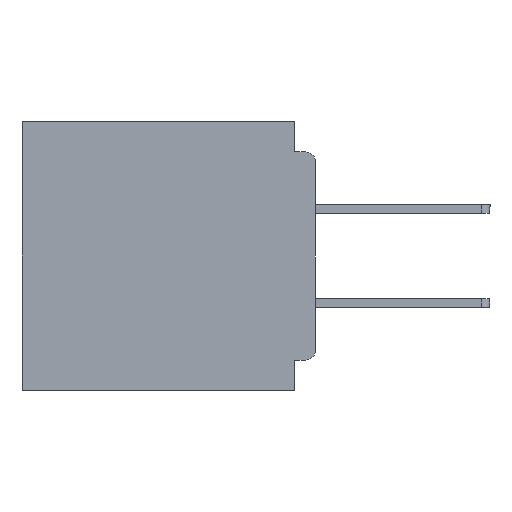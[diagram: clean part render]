
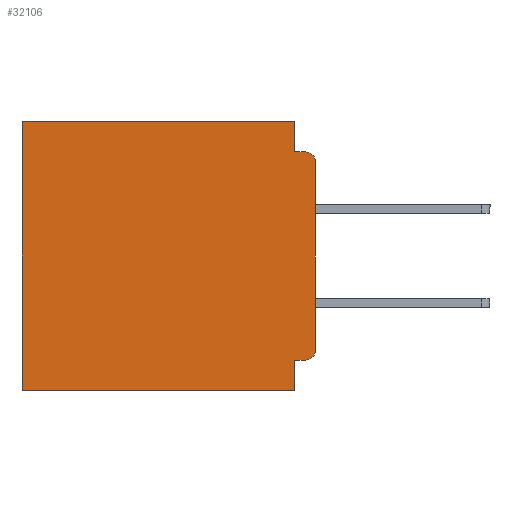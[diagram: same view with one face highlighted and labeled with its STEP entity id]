
A CAD part, left-side view. The second image highlights one B-rep face of the part: STEP entity #32106.
In plain terms, the highlighted planar face has unit normal (-1, 0, 0).
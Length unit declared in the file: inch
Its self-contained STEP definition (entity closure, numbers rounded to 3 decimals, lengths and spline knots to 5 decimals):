
#541 = LINE ( 'NONE', #1973, #42620 ) ;
#576 = EDGE_CURVE ( 'NONE', #24921, #27459, #48411, .T. ) ;
#1276 = VERTEX_POINT ( 'NONE', #49345 ) ;
#1973 = CARTESIAN_POINT ( 'NONE',  ( 0.3, 0., -0.4 ) ) ;
#2923 = ORIENTED_EDGE ( 'NONE', *, *, #19662, .F. ) ;
#3037 = ORIENTED_EDGE ( 'NONE', *, *, #3956, .F. ) ;
#3356 = EDGE_CURVE ( 'NONE', #4445, #14163, #34812, .T. ) ;
#3956 = EDGE_CURVE ( 'NONE', #1276, #4445, #29619, .T. ) ;
#4445 = VERTEX_POINT ( 'NONE', #17916 ) ;
#4717 = CARTESIAN_POINT ( 'NONE',  ( 0.3, 0., -0.4 ) ) ;
#5604 = ORIENTED_EDGE ( 'NONE', *, *, #14906, .F. ) ;
#8068 = ORIENTED_EDGE ( 'NONE', *, *, #576, .F. ) ;
#8786 = DIRECTION ( 'NONE',  ( 1., 0., 0. ) ) ;
#9751 = CIRCLE ( 'NONE', #35528, 0.015 ) ;
#9916 = ORIENTED_EDGE ( 'NONE', *, *, #21294, .T. ) ;
#10152 = CARTESIAN_POINT ( 'NONE',  ( 0.3, 0.437, 0. ) ) ;
#10238 = CARTESIAN_POINT ( 'NONE',  ( 0.3, 0.031, -0.4 ) ) ;
#14163 = VERTEX_POINT ( 'NONE', #17513 ) ;
#14285 = ORIENTED_EDGE ( 'NONE', *, *, #16087, .T. ) ;
#14349 = CARTESIAN_POINT ( 'NONE',  ( 0.3, 0., -0.045 ) ) ;
#14906 = EDGE_CURVE ( 'NONE', #37538, #44728, #541, .T. ) ;
#15687 = CARTESIAN_POINT ( 'NONE',  ( 0.3, 0., -0.355 ) ) ;
#15803 = LINE ( 'NONE', #40342, #40226 ) ;
#16087 = EDGE_CURVE ( 'NONE', #18767, #38620, #46026, .T. ) ;
#17513 = CARTESIAN_POINT ( 'NONE',  ( 0.3, 0.015, -0.045 ) ) ;
#17916 = CARTESIAN_POINT ( 'NONE',  ( 0.3, 0.031, -0.045 ) ) ;
#18767 = VERTEX_POINT ( 'NONE', #10152 ) ;
#19227 = CARTESIAN_POINT ( 'NONE',  ( 0.3, 0.015, -0.06 ) ) ;
#19255 = DIRECTION ( 'NONE',  ( 0., 1., 0. ) ) ;
#19662 = EDGE_CURVE ( 'NONE', #27459, #32851, #29667, .T. ) ;
#19992 = DIRECTION ( 'NONE',  ( 0., 1., 0. ) ) ;
#21294 = EDGE_CURVE ( 'NONE', #1276, #18767, #33327, .T. ) ;
#22009 = CARTESIAN_POINT ( 'NONE',  ( 0.3, 0., -0.34 ) ) ;
#22091 = DIRECTION ( 'NONE',  ( 0., 1., 0. ) ) ;
#22133 = CARTESIAN_POINT ( 'NONE',  ( 0.3, 0.437, -0.4 ) ) ;
#22221 = CARTESIAN_POINT ( 'NONE',  ( 0.3, 0.031, -0.355 ) ) ;
#22444 = VECTOR ( 'NONE', #19255, 39.37008 ) ;
#22645 = CARTESIAN_POINT ( 'NONE',  ( 0.3, 0.015, -0.34 ) ) ;
#22954 = CARTESIAN_POINT ( 'NONE',  ( 0.3, 0.031, 0. ) ) ;
#23049 = VECTOR ( 'NONE', #30181, 39.37008 ) ;
#23368 = ORIENTED_EDGE ( 'NONE', *, *, #3356, .F. ) ;
#23937 = VECTOR ( 'NONE', #33295, 39.37008 ) ;
#24040 = DIRECTION ( 'NONE',  ( 0., 0., -1. ) ) ;
#24921 = VERTEX_POINT ( 'NONE', #25912 ) ;
#25865 = ORIENTED_EDGE ( 'NONE', *, *, #41685, .T. ) ;
#25912 = CARTESIAN_POINT ( 'NONE',  ( 0.3, 0.015, -0.355 ) ) ;
#26760 = DIRECTION ( 'NONE',  ( 0., 0., -1. ) ) ;
#27459 = VERTEX_POINT ( 'NONE', #22221 ) ;
#29060 = PLANE ( 'NONE',  #47614 ) ;
#29619 = LINE ( 'NONE', #22954, #37915 ) ;
#29667 = LINE ( 'NONE', #40519, #51283 ) ;
#30181 = DIRECTION ( 'NONE',  ( 0., 0., -1. ) ) ;
#30219 = EDGE_LOOP ( 'NONE', ( #5604, #38073, #23368, #3037, #9916, #14285, #32913, #2923, #8068, #25865 ) ) ;
#32106 = ADVANCED_FACE ( 'NONE', ( #40430 ), #29060, .F. ) ;
#32851 = VERTEX_POINT ( 'NONE', #10238 ) ;
#32913 = ORIENTED_EDGE ( 'NONE', *, *, #40198, .F. ) ;
#33295 = DIRECTION ( 'NONE',  ( 0., -1., 0. ) ) ;
#33327 = LINE ( 'NONE', #39599, #22444 ) ;
#34812 = LINE ( 'NONE', #14349, #23937 ) ;
#35528 = AXIS2_PLACEMENT_3D ( 'NONE', #19227, #47730, #24040 ) ;
#37302 = DIRECTION ( 'NONE',  ( 0., 0., -1. ) ) ;
#37538 = VERTEX_POINT ( 'NONE', #42767 ) ;
#37591 = VECTOR ( 'NONE', #22091, 39.37008 ) ;
#37644 = EDGE_CURVE ( 'NONE', #37538, #14163, #9751, .T. ) ;
#37915 = VECTOR ( 'NONE', #51402, 39.37008 ) ;
#38073 = ORIENTED_EDGE ( 'NONE', *, *, #37644, .T. ) ;
#38620 = VERTEX_POINT ( 'NONE', #45977 ) ;
#38822 = CIRCLE ( 'NONE', #51974, 0.015 ) ;
#39599 = CARTESIAN_POINT ( 'NONE',  ( 0.3, 0., 0. ) ) ;
#40198 = EDGE_CURVE ( 'NONE', #32851, #38620, #15803, .T. ) ;
#40226 = VECTOR ( 'NONE', #19992, 39.37008 ) ;
#40342 = CARTESIAN_POINT ( 'NONE',  ( 0.3, 0., -0.4 ) ) ;
#40430 = FACE_OUTER_BOUND ( 'NONE', #30219, .T. ) ;
#40519 = CARTESIAN_POINT ( 'NONE',  ( 0.3, 0.031, -0.4 ) ) ;
#41685 = EDGE_CURVE ( 'NONE', #24921, #44728, #38822, .T. ) ;
#42620 = VECTOR ( 'NONE', #42747, 39.37008 ) ;
#42747 = DIRECTION ( 'NONE',  ( 0., 0., -1. ) ) ;
#42767 = CARTESIAN_POINT ( 'NONE',  ( 0.3, 0., -0.06 ) ) ;
#44728 = VERTEX_POINT ( 'NONE', #22009 ) ;
#45977 = CARTESIAN_POINT ( 'NONE',  ( 0.3, 0.437, -0.4 ) ) ;
#46026 = LINE ( 'NONE', #22133, #23049 ) ;
#47614 = AXIS2_PLACEMENT_3D ( 'NONE', #4717, #8786, #37302 ) ;
#47730 = DIRECTION ( 'NONE',  ( -1., 0., 0. ) ) ;
#48411 = LINE ( 'NONE', #15687, #37591 ) ;
#49345 = CARTESIAN_POINT ( 'NONE',  ( 0.3, 0.031, 0. ) ) ;
#51095 = DIRECTION ( 'NONE',  ( -1., 0., 0. ) ) ;
#51283 = VECTOR ( 'NONE', #52679, 39.37008 ) ;
#51402 = DIRECTION ( 'NONE',  ( 0., 0., -1. ) ) ;
#51974 = AXIS2_PLACEMENT_3D ( 'NONE', #22645, #51095, #26760 ) ;
#52679 = DIRECTION ( 'NONE',  ( 0., 0., -1. ) ) ;
